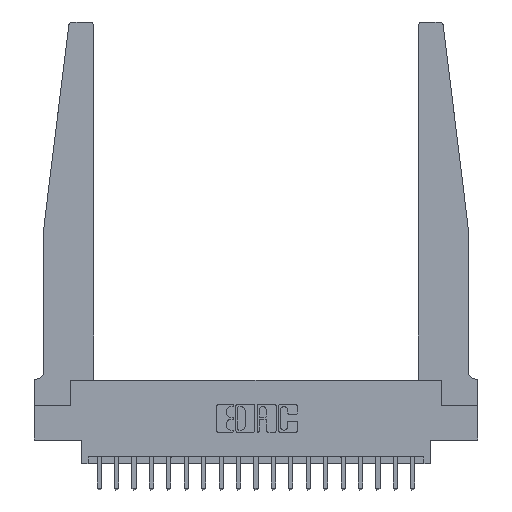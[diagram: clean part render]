
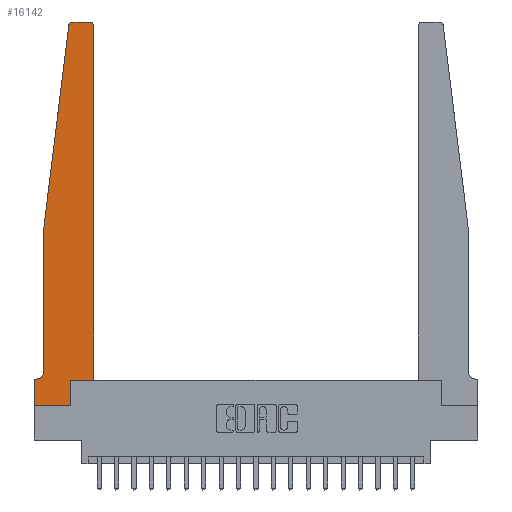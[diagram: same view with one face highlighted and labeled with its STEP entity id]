
A CAD part, top view. The second image highlights one B-rep face of the part: STEP entity #16142.
In plain terms, the highlighted planar face has unit normal (0, 0, 1).
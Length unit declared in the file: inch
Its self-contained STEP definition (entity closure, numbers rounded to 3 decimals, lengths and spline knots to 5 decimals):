
#236 = LINE ( 'NONE', #6887, #16593 ) ;
#255 = CARTESIAN_POINT ( 'NONE',  ( 0.065, 1.25, 0.37 ) ) ;
#431 = DIRECTION ( 'NONE',  ( 0., -1., 0. ) ) ;
#556 = DIRECTION ( 'NONE',  ( 0., 1., 0. ) ) ;
#626 = EDGE_CURVE ( 'NONE', #4580, #1143, #10017, .T. ) ;
#938 = ORIENTED_EDGE ( 'NONE', *, *, #2830, .T. ) ;
#1143 = VERTEX_POINT ( 'NONE', #13873 ) ;
#1507 = LINE ( 'NONE', #10478, #10473 ) ;
#1794 = CARTESIAN_POINT ( 'NONE',  ( 0.065, 0.1875, 0.37 ) ) ;
#1820 = DIRECTION ( 'NONE',  ( 0., 0., -1. ) ) ;
#1891 = LINE ( 'NONE', #1794, #18249 ) ;
#1935 = LINE ( 'NONE', #8490, #14105 ) ;
#1943 = CARTESIAN_POINT ( 'NONE',  ( 0.2605, 0.18, 0.37 ) ) ;
#2006 = CARTESIAN_POINT ( 'NONE',  ( 0.425, 0.18, 0.37 ) ) ;
#2147 = VERTEX_POINT ( 'NONE', #255 ) ;
#2319 = VERTEX_POINT ( 'NONE', #13424 ) ;
#2830 = EDGE_CURVE ( 'NONE', #2147, #2319, #13895, .T. ) ;
#2910 = EDGE_CURVE ( 'NONE', #16735, #13291, #236, .T. ) ;
#2921 = LINE ( 'NONE', #2006, #15084 ) ;
#3335 = VERTEX_POINT ( 'NONE', #11042 ) ;
#4011 = CARTESIAN_POINT ( 'NONE',  ( 0., 0., 0.37 ) ) ;
#4126 = CARTESIAN_POINT ( 'NONE',  ( 0.395, 2.72, 0.37 ) ) ;
#4169 = ORIENTED_EDGE ( 'NONE', *, *, #12785, .T. ) ;
#4580 = VERTEX_POINT ( 'NONE', #18256 ) ;
#5134 = DIRECTION ( 'NONE',  ( 0., 0., 1. ) ) ;
#5159 = ORIENTED_EDGE ( 'NONE', *, *, #16906, .T. ) ;
#5216 = DIRECTION ( 'NONE',  ( 1., 0., 0. ) ) ;
#5488 = CARTESIAN_POINT ( 'NONE',  ( 0.25, 2.75, 0.37 ) ) ;
#5633 = CARTESIAN_POINT ( 'NONE',  ( 0., 0., 0.37 ) ) ;
#5758 = DIRECTION ( 'NONE',  ( 1., 0., 0. ) ) ;
#5784 = VECTOR ( 'NONE', #18162, 39.37008 ) ;
#5871 = VERTEX_POINT ( 'NONE', #8819 ) ;
#5959 = VERTEX_POINT ( 'NONE', #14072 ) ;
#6153 = CARTESIAN_POINT ( 'NONE',  ( 0., 0.1875, 0.37 ) ) ;
#6297 = ORIENTED_EDGE ( 'NONE', *, *, #9557, .T. ) ;
#6669 = VERTEX_POINT ( 'NONE', #6153 ) ;
#6887 = CARTESIAN_POINT ( 'NONE',  ( 0.2605, 0.18, 0.37 ) ) ;
#7260 = DIRECTION ( 'NONE',  ( 1., 0., 0. ) ) ;
#7641 = EDGE_CURVE ( 'NONE', #3335, #16735, #14286, .T. ) ;
#8060 = EDGE_CURVE ( 'NONE', #6669, #3335, #11065, .T. ) ;
#8353 = DIRECTION ( 'NONE',  ( 1., 0., 0. ) ) ;
#8490 = CARTESIAN_POINT ( 'NONE',  ( 0.425, 0.18, 0.37 ) ) ;
#8819 = CARTESIAN_POINT ( 'NONE',  ( 0.425, 2.72, 0.37 ) ) ;
#9119 = VERTEX_POINT ( 'NONE', #10179 ) ;
#9147 = ORIENTED_EDGE ( 'NONE', *, *, #15380, .T. ) ;
#9271 = AXIS2_PLACEMENT_3D ( 'NONE', #4126, #15245, #5758 ) ;
#9557 = EDGE_CURVE ( 'NONE', #2319, #15181, #9804, .T. ) ;
#9804 = CIRCLE ( 'NONE', #11827, 0.05 ) ;
#9957 = CARTESIAN_POINT ( 'NONE',  ( 0.065, 1.25, 0.37 ) ) ;
#10017 = LINE ( 'NONE', #5488, #5784 ) ;
#10077 = DIRECTION ( 'NONE',  ( 0., 1., 0. ) ) ;
#10179 = CARTESIAN_POINT ( 'NONE',  ( 0.24675, 2.72367, 0.37 ) ) ;
#10236 = ORIENTED_EDGE ( 'NONE', *, *, #13287, .T. ) ;
#10473 = VECTOR ( 'NONE', #16843, 39.37008 ) ;
#10478 = CARTESIAN_POINT ( 'NONE',  ( 0.065, 1.25, 0.37 ) ) ;
#11042 = CARTESIAN_POINT ( 'NONE',  ( 0., 0., 0.37 ) ) ;
#11065 = LINE ( 'NONE', #5633, #14740 ) ;
#11328 = DIRECTION ( 'NONE',  ( -1., 0., 0. ) ) ;
#11349 = CARTESIAN_POINT ( 'NONE',  ( 0.015, 0.2375, 0.37 ) ) ;
#11357 = EDGE_LOOP ( 'NONE', ( #13916, #10236, #5159, #938, #6297, #4169, #18672, #16326, #17343, #16229, #18981, #9147 ) ) ;
#11558 = PLANE ( 'NONE',  #14816 ) ;
#11608 = CARTESIAN_POINT ( 'NONE',  ( 0.015, 0.1875, 0.37 ) ) ;
#11827 = AXIS2_PLACEMENT_3D ( 'NONE', #11349, #1820, #12931 ) ;
#12785 = EDGE_CURVE ( 'NONE', #15181, #6669, #1891, .T. ) ;
#12931 = DIRECTION ( 'NONE',  ( -1., 0., 0. ) ) ;
#13151 = CARTESIAN_POINT ( 'NONE',  ( 0., 0.1875, 0.37 ) ) ;
#13248 = CARTESIAN_POINT ( 'NONE',  ( 0.2605, 0., 0.37 ) ) ;
#13287 = EDGE_CURVE ( 'NONE', #1143, #9119, #15004, .T. ) ;
#13291 = VERTEX_POINT ( 'NONE', #1943 ) ;
#13424 = CARTESIAN_POINT ( 'NONE',  ( 0.065, 0.2375, 0.37 ) ) ;
#13458 = CIRCLE ( 'NONE', #9271, 0.03 ) ;
#13873 = CARTESIAN_POINT ( 'NONE',  ( 0.27653, 2.75, 0.37 ) ) ;
#13895 = LINE ( 'NONE', #9957, #14375 ) ;
#13916 = ORIENTED_EDGE ( 'NONE', *, *, #626, .T. ) ;
#14072 = CARTESIAN_POINT ( 'NONE',  ( 0.425, 0.18, 0.37 ) ) ;
#14105 = VECTOR ( 'NONE', #556, 39.37008 ) ;
#14286 = LINE ( 'NONE', #4011, #17519 ) ;
#14375 = VECTOR ( 'NONE', #431, 39.37008 ) ;
#14622 = CARTESIAN_POINT ( 'NONE',  ( 0.27653, 2.72, 0.37 ) ) ;
#14709 = DIRECTION ( 'NONE',  ( 0., 0., 1. ) ) ;
#14740 = VECTOR ( 'NONE', #18303, 39.37008 ) ;
#14816 = AXIS2_PLACEMENT_3D ( 'NONE', #13151, #14709, #5216 ) ;
#15004 = CIRCLE ( 'NONE', #17049, 0.03 ) ;
#15084 = VECTOR ( 'NONE', #8353, 39.37008 ) ;
#15181 = VERTEX_POINT ( 'NONE', #11608 ) ;
#15245 = DIRECTION ( 'NONE',  ( 0., 0., 1. ) ) ;
#15380 = EDGE_CURVE ( 'NONE', #5871, #4580, #13458, .T. ) ;
#16142 = ADVANCED_FACE ( 'NONE', ( #18156 ), #11558, .T. ) ;
#16229 = ORIENTED_EDGE ( 'NONE', *, *, #18635, .T. ) ;
#16231 = DIRECTION ( 'NONE',  ( 1., 0., 0. ) ) ;
#16326 = ORIENTED_EDGE ( 'NONE', *, *, #7641, .T. ) ;
#16593 = VECTOR ( 'NONE', #10077, 39.37008 ) ;
#16735 = VERTEX_POINT ( 'NONE', #13248 ) ;
#16843 = DIRECTION ( 'NONE',  ( -0.122, -0.992, 0. ) ) ;
#16906 = EDGE_CURVE ( 'NONE', #9119, #2147, #1507, .T. ) ;
#17049 = AXIS2_PLACEMENT_3D ( 'NONE', #14622, #5134, #16231 ) ;
#17343 = ORIENTED_EDGE ( 'NONE', *, *, #2910, .T. ) ;
#17519 = VECTOR ( 'NONE', #7260, 39.37008 ) ;
#18156 = FACE_OUTER_BOUND ( 'NONE', #11357, .T. ) ;
#18162 = DIRECTION ( 'NONE',  ( -1., 0., 0. ) ) ;
#18249 = VECTOR ( 'NONE', #11328, 39.37008 ) ;
#18256 = CARTESIAN_POINT ( 'NONE',  ( 0.395, 2.75, 0.37 ) ) ;
#18303 = DIRECTION ( 'NONE',  ( 0., -1., 0. ) ) ;
#18635 = EDGE_CURVE ( 'NONE', #13291, #5959, #2921, .T. ) ;
#18670 = EDGE_CURVE ( 'NONE', #5959, #5871, #1935, .T. ) ;
#18672 = ORIENTED_EDGE ( 'NONE', *, *, #8060, .T. ) ;
#18981 = ORIENTED_EDGE ( 'NONE', *, *, #18670, .T. ) ;
